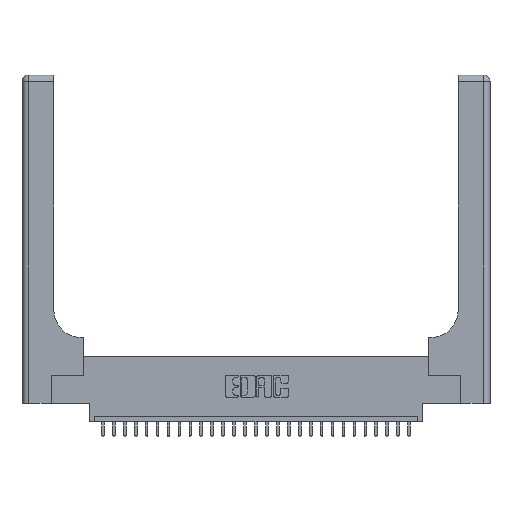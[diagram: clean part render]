
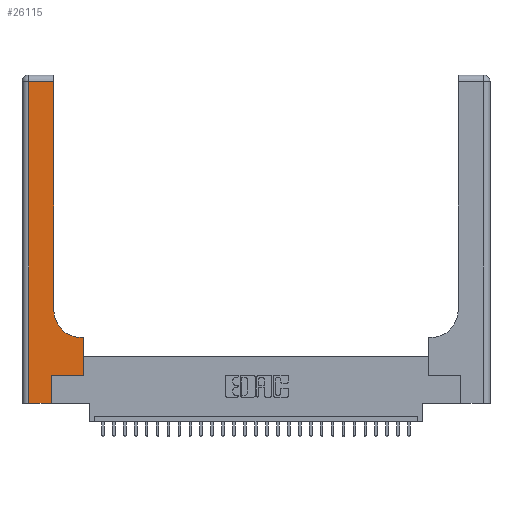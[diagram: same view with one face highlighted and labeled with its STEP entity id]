
A CAD part, top view. The second image highlights one B-rep face of the part: STEP entity #26115.
In plain terms, the highlighted planar face has unit normal (0, 0, 1).
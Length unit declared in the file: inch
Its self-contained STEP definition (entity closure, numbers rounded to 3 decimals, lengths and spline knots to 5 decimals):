
#1109 = DIRECTION ( 'NONE',  ( 1., 0., 0. ) ) ;
#1495 = DIRECTION ( 'NONE',  ( 1., 0., 0. ) ) ;
#1521 = CARTESIAN_POINT ( 'NONE',  ( 0.5415, 0.6, 0.37 ) ) ;
#2188 = VECTOR ( 'NONE', #25788, 39.37008 ) ;
#2664 = VERTEX_POINT ( 'NONE', #3711 ) ;
#2903 = LINE ( 'NONE', #22145, #27332 ) ;
#3009 = LINE ( 'NONE', #6916, #23271 ) ;
#3711 = CARTESIAN_POINT ( 'NONE',  ( 0.2915, 2.94, 0.37 ) ) ;
#3751 = DIRECTION ( 'NONE',  ( 0., 0., -1. ) ) ;
#3843 = VERTEX_POINT ( 'NONE', #7325 ) ;
#4163 = CARTESIAN_POINT ( 'NONE',  ( 0.2915, 0.85, 0.37 ) ) ;
#4235 = LINE ( 'NONE', #19201, #18914 ) ;
#4348 = ORIENTED_EDGE ( 'NONE', *, *, #17766, .T. ) ;
#4696 = VERTEX_POINT ( 'NONE', #16313 ) ;
#6290 = CARTESIAN_POINT ( 'NONE',  ( 0.5415, 0.85, 0.37 ) ) ;
#6590 = EDGE_CURVE ( 'NONE', #3843, #22405, #4235, .T. ) ;
#6916 = CARTESIAN_POINT ( 'NONE',  ( 0.2915, 0.6, 0.37 ) ) ;
#7014 = CARTESIAN_POINT ( 'NONE',  ( 0.06, 2.94, 0.37 ) ) ;
#7325 = CARTESIAN_POINT ( 'NONE',  ( 0.269, 0.25, 0.37 ) ) ;
#7679 = CARTESIAN_POINT ( 'NONE',  ( 0.269, 0., 0.37 ) ) ;
#8149 = LINE ( 'NONE', #10215, #2188 ) ;
#8732 = VECTOR ( 'NONE', #12114, 39.37008 ) ;
#8773 = ORIENTED_EDGE ( 'NONE', *, *, #6590, .T. ) ;
#8839 = PLANE ( 'NONE',  #16755 ) ;
#9052 = LINE ( 'NONE', #24531, #18806 ) ;
#9060 = ORIENTED_EDGE ( 'NONE', *, *, #24399, .T. ) ;
#9332 = VECTOR ( 'NONE', #22690, 39.37008 ) ;
#9439 = LINE ( 'NONE', #21085, #8732 ) ;
#9513 = CARTESIAN_POINT ( 'NONE',  ( 0.06, 3., 0.37 ) ) ;
#10215 = CARTESIAN_POINT ( 'NONE',  ( 0.5585, 0.25, 0.37 ) ) ;
#10267 = EDGE_LOOP ( 'NONE', ( #20005, #23300, #4348, #22469, #22812, #8773, #12964, #13062, #9060 ) ) ;
#11034 = VECTOR ( 'NONE', #15925, 39.37008 ) ;
#11123 = CARTESIAN_POINT ( 'NONE',  ( 0.5585, 0.6, 0.37 ) ) ;
#11715 = VERTEX_POINT ( 'NONE', #7679 ) ;
#12114 = DIRECTION ( 'NONE',  ( 0., 1., 0. ) ) ;
#12964 = ORIENTED_EDGE ( 'NONE', *, *, #28818, .T. ) ;
#13062 = ORIENTED_EDGE ( 'NONE', *, *, #18136, .T. ) ;
#13325 = CARTESIAN_POINT ( 'NONE',  ( 0., 3., 0.37 ) ) ;
#13532 = LINE ( 'NONE', #9513, #9332 ) ;
#15285 = DIRECTION ( 'NONE',  ( -1., 0., 0. ) ) ;
#15541 = DIRECTION ( 'NONE',  ( 0., 0., -1. ) ) ;
#15925 = DIRECTION ( 'NONE',  ( 1., 0., 0. ) ) ;
#16128 = VERTEX_POINT ( 'NONE', #1521 ) ;
#16313 = CARTESIAN_POINT ( 'NONE',  ( 0.06, 0., 0.37 ) ) ;
#16755 = AXIS2_PLACEMENT_3D ( 'NONE', #13325, #15541, #26932 ) ;
#17766 = EDGE_CURVE ( 'NONE', #20283, #4696, #13532, .T. ) ;
#17967 = CIRCLE ( 'NONE', #22933, 0.25 ) ;
#18136 = EDGE_CURVE ( 'NONE', #20709, #16128, #3009, .T. ) ;
#18806 = VECTOR ( 'NONE', #15285, 39.37008 ) ;
#18914 = VECTOR ( 'NONE', #1109, 39.37008 ) ;
#19201 = CARTESIAN_POINT ( 'NONE',  ( 0.269, 0.25, 0.37 ) ) ;
#19582 = EDGE_CURVE ( 'NONE', #4696, #11715, #19766, .T. ) ;
#19766 = LINE ( 'NONE', #24719, #11034 ) ;
#19804 = DIRECTION ( 'NONE',  ( 0., 1., 0. ) ) ;
#20005 = ORIENTED_EDGE ( 'NONE', *, *, #21508, .T. ) ;
#20283 = VERTEX_POINT ( 'NONE', #7014 ) ;
#20505 = EDGE_CURVE ( 'NONE', #11715, #3843, #2903, .T. ) ;
#20567 = VERTEX_POINT ( 'NONE', #4163 ) ;
#20709 = VERTEX_POINT ( 'NONE', #11123 ) ;
#21085 = CARTESIAN_POINT ( 'NONE',  ( 0.2915, 3., 0.37 ) ) ;
#21508 = EDGE_CURVE ( 'NONE', #20567, #2664, #9439, .T. ) ;
#22145 = CARTESIAN_POINT ( 'NONE',  ( 0.269, 0., 0.37 ) ) ;
#22279 = EDGE_CURVE ( 'NONE', #2664, #20283, #9052, .T. ) ;
#22316 = CARTESIAN_POINT ( 'NONE',  ( 0.5585, 0.25, 0.37 ) ) ;
#22405 = VERTEX_POINT ( 'NONE', #22316 ) ;
#22469 = ORIENTED_EDGE ( 'NONE', *, *, #19582, .T. ) ;
#22690 = DIRECTION ( 'NONE',  ( 0., -1., 0. ) ) ;
#22732 = DIRECTION ( 'NONE',  ( -1., 0., 0. ) ) ;
#22812 = ORIENTED_EDGE ( 'NONE', *, *, #20505, .T. ) ;
#22933 = AXIS2_PLACEMENT_3D ( 'NONE', #6290, #3751, #1495 ) ;
#23271 = VECTOR ( 'NONE', #22732, 39.37008 ) ;
#23300 = ORIENTED_EDGE ( 'NONE', *, *, #22279, .T. ) ;
#24399 = EDGE_CURVE ( 'NONE', #16128, #20567, #17967, .T. ) ;
#24531 = CARTESIAN_POINT ( 'NONE',  ( 0., 2.94, 0.37 ) ) ;
#24719 = CARTESIAN_POINT ( 'NONE',  ( 0., 0., 0.37 ) ) ;
#25557 = FACE_OUTER_BOUND ( 'NONE', #10267, .T. ) ;
#25788 = DIRECTION ( 'NONE',  ( 0., 1., 0. ) ) ;
#26115 = ADVANCED_FACE ( 'NONE', ( #25557 ), #8839, .F. ) ;
#26932 = DIRECTION ( 'NONE',  ( -1., 0., 0. ) ) ;
#27332 = VECTOR ( 'NONE', #19804, 39.37008 ) ;
#28818 = EDGE_CURVE ( 'NONE', #22405, #20709, #8149, .T. ) ;
